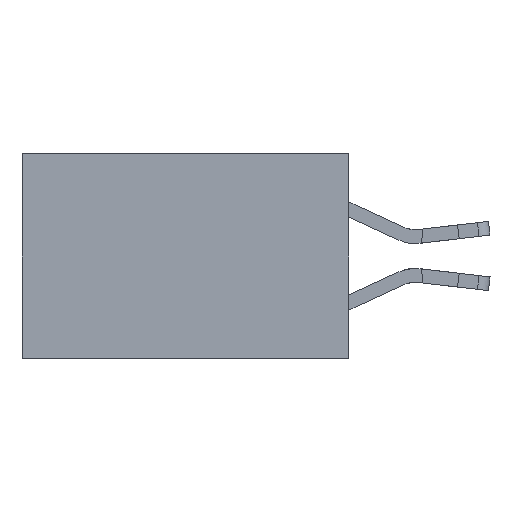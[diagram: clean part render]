
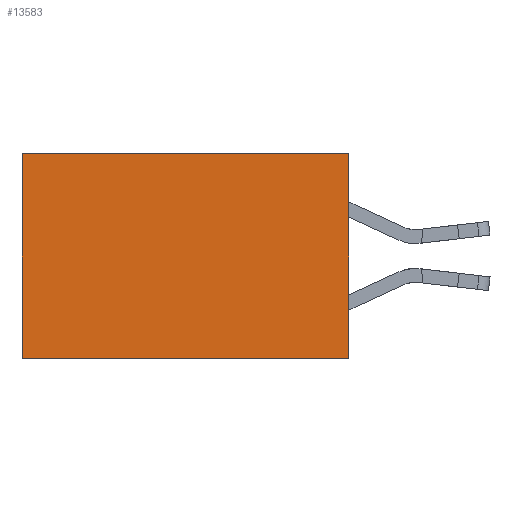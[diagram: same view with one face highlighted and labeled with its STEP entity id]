
A CAD part, left-side view. The second image highlights one B-rep face of the part: STEP entity #13583.
In plain terms, the highlighted planar face has unit normal (-1, 0, 0).
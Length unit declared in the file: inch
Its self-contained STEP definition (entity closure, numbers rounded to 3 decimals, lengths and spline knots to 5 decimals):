
#1157 = CARTESIAN_POINT ( 'NONE',  ( 0.277, 0., -0.37 ) ) ;
#1213 = DIRECTION ( 'NONE',  ( 0., 0., -1. ) ) ;
#1635 = VECTOR ( 'NONE', #19904, 39.37008 ) ;
#4594 = AXIS2_PLACEMENT_3D ( 'NONE', #13571, #29313, #15855 ) ;
#4621 = CARTESIAN_POINT ( 'NONE',  ( 0.277, 0., -0.37 ) ) ;
#5076 = VERTEX_POINT ( 'NONE', #18591 ) ;
#5167 = DIRECTION ( 'NONE',  ( 0., 1., 0. ) ) ;
#5416 = LINE ( 'NONE', #4621, #10789 ) ;
#5485 = EDGE_CURVE ( 'NONE', #5076, #10298, #5416, .T. ) ;
#5670 = LINE ( 'NONE', #1157, #11048 ) ;
#5827 = EDGE_LOOP ( 'NONE', ( #17849, #27843, #12306, #6347 ) ) ;
#6347 = ORIENTED_EDGE ( 'NONE', *, *, #21249, .T. ) ;
#7083 = EDGE_CURVE ( 'NONE', #27605, #5076, #5670, .T. ) ;
#9293 = VECTOR ( 'NONE', #26896, 39.37008 ) ;
#10298 = VERTEX_POINT ( 'NONE', #20695 ) ;
#10789 = VECTOR ( 'NONE', #5167, 39.37008 ) ;
#11048 = VECTOR ( 'NONE', #1213, 39.37008 ) ;
#11088 = CARTESIAN_POINT ( 'NONE',  ( 0.277, 0., 0. ) ) ;
#12306 = ORIENTED_EDGE ( 'NONE', *, *, #7083, .F. ) ;
#12509 = VERTEX_POINT ( 'NONE', #25822 ) ;
#13571 = CARTESIAN_POINT ( 'NONE',  ( 0.277, 0., -0.37 ) ) ;
#13583 = ADVANCED_FACE ( 'NONE', ( #21877 ), #22550, .F. ) ;
#13944 = LINE ( 'NONE', #17663, #1635 ) ;
#15855 = DIRECTION ( 'NONE',  ( 0., 0., -1. ) ) ;
#17663 = CARTESIAN_POINT ( 'NONE',  ( 0.277, 0.59, -0.37 ) ) ;
#17849 = ORIENTED_EDGE ( 'NONE', *, *, #28626, .T. ) ;
#18591 = CARTESIAN_POINT ( 'NONE',  ( 0.277, 0., -0.37 ) ) ;
#19904 = DIRECTION ( 'NONE',  ( 0., 0., -1. ) ) ;
#20695 = CARTESIAN_POINT ( 'NONE',  ( 0.277, 0.59, -0.37 ) ) ;
#21249 = EDGE_CURVE ( 'NONE', #27605, #12509, #26633, .T. ) ;
#21877 = FACE_OUTER_BOUND ( 'NONE', #5827, .T. ) ;
#22550 = PLANE ( 'NONE',  #4594 ) ;
#25822 = CARTESIAN_POINT ( 'NONE',  ( 0.277, 0.59, 0. ) ) ;
#25892 = CARTESIAN_POINT ( 'NONE',  ( 0.277, 0., 0. ) ) ;
#26633 = LINE ( 'NONE', #11088, #9293 ) ;
#26896 = DIRECTION ( 'NONE',  ( 0., 1., 0. ) ) ;
#27605 = VERTEX_POINT ( 'NONE', #25892 ) ;
#27843 = ORIENTED_EDGE ( 'NONE', *, *, #5485, .F. ) ;
#28626 = EDGE_CURVE ( 'NONE', #12509, #10298, #13944, .T. ) ;
#29313 = DIRECTION ( 'NONE',  ( 1., 0., 0. ) ) ;
